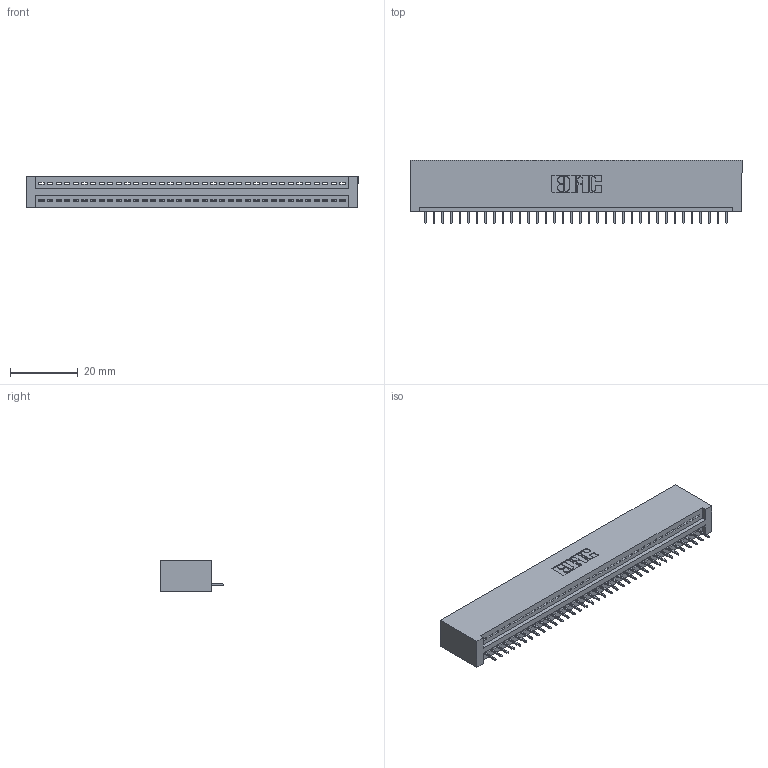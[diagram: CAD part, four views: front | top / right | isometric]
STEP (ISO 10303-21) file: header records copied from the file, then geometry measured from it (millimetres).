
FILE_DESCRIPTION (( 'STEP AP203' ), '1' );
FILE_NAME ('395-036-525-101.STEP', '2020-09-23T23:18:15', ( '' ), ( '' ), 'SwSTEP 2.0', 'SolidWorks 2020', '' );
FILE_SCHEMA (( 'CONFIG_CONTROL_DESIGN' ));
Length unit declared in the file: inch
Products named in the file (3): 345-292-001_345-293-125; 395-036-525-101; 345 Part_No Mounting Lugs
Assembly tree (37 placements, depth 2):
  395-036-525-101
    345 Part_No Mounting Lugs
    345-292-001_345-293-125  x36
Bounding box: 98.04 x 18.72 x 9.4 mm (x, y, z)
Volume: 9700.5 mm3; surface area: 12509.6 mm2
Topology: 37 solids, 37 shells, 2350 faces, 6797 edges, 4386 vertices
Faces by surface type: plane 1732, cylinder 618
Entity records: 27699 total; most frequent: CARTESIAN_POINT 4804, ORIENTED_EDGE 4774, DIRECTION 4199, EDGE_CURVE 2387, VECTOR 2123, LINE 2123, VERTEX_POINT 1586, AXIS2_PLACEMENT_3D 1038
